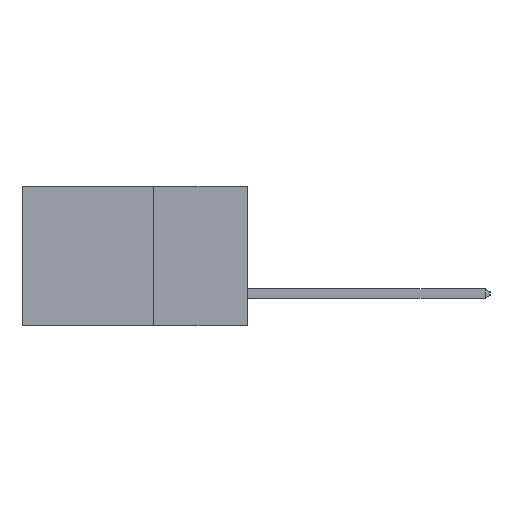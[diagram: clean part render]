
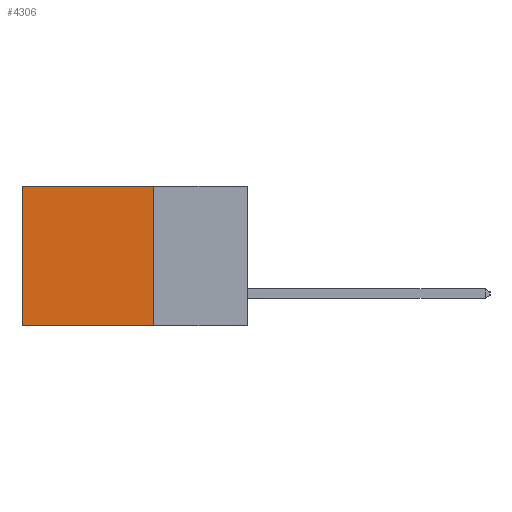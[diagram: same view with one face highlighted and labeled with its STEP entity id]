
A CAD part, left-side view. The second image highlights one B-rep face of the part: STEP entity #4306.
In plain terms, the highlighted planar face has unit normal (-1, 0, 0).
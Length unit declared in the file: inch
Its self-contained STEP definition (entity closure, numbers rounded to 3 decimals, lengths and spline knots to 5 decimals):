
#258 = FACE_OUTER_BOUND ( 'NONE', #11294, .T. ) ;
#432 = ORIENTED_EDGE ( 'NONE', *, *, #4121, .T. ) ;
#557 = VECTOR ( 'NONE', #14478, 39.37008 ) ;
#993 = LINE ( 'NONE', #14467, #557 ) ;
#1541 = VERTEX_POINT ( 'NONE', #5240 ) ;
#1829 = VECTOR ( 'NONE', #15657, 39.37008 ) ;
#1896 = CARTESIAN_POINT ( 'NONE',  ( 0.298, 0.25, 0. ) ) ;
#2650 = CARTESIAN_POINT ( 'NONE',  ( 0.298, 0.6, -0.37 ) ) ;
#3651 = VERTEX_POINT ( 'NONE', #2650 ) ;
#3961 = EDGE_CURVE ( 'NONE', #1541, #5538, #9149, .T. ) ;
#4121 = EDGE_CURVE ( 'NONE', #1541, #4907, #9777, .T. ) ;
#4306 = ADVANCED_FACE ( 'NONE', ( #258 ), #14654, .F. ) ;
#4907 = VERTEX_POINT ( 'NONE', #16112 ) ;
#4939 = VECTOR ( 'NONE', #8704, 39.37008 ) ;
#5240 = CARTESIAN_POINT ( 'NONE',  ( 0.298, 0.25, 0. ) ) ;
#5258 = EDGE_CURVE ( 'NONE', #5538, #3651, #12749, .T. ) ;
#5538 = VERTEX_POINT ( 'NONE', #16472 ) ;
#5621 = ORIENTED_EDGE ( 'NONE', *, *, #5258, .F. ) ;
#6092 = VECTOR ( 'NONE', #14406, 39.37008 ) ;
#6339 = EDGE_CURVE ( 'NONE', #4907, #3651, #993, .T. ) ;
#7039 = AXIS2_PLACEMENT_3D ( 'NONE', #8449, #14758, #12980 ) ;
#7514 = ORIENTED_EDGE ( 'NONE', *, *, #6339, .T. ) ;
#8449 = CARTESIAN_POINT ( 'NONE',  ( 0.298, 0.25, 0. ) ) ;
#8704 = DIRECTION ( 'NONE',  ( 0., 1., 0. ) ) ;
#9149 = LINE ( 'NONE', #16327, #1829 ) ;
#9777 = LINE ( 'NONE', #1896, #6092 ) ;
#11294 = EDGE_LOOP ( 'NONE', ( #7514, #5621, #14216, #432 ) ) ;
#12749 = LINE ( 'NONE', #13396, #4939 ) ;
#12980 = DIRECTION ( 'NONE',  ( 0., 0., -1. ) ) ;
#13396 = CARTESIAN_POINT ( 'NONE',  ( 0.298, 0.25, -0.37 ) ) ;
#14216 = ORIENTED_EDGE ( 'NONE', *, *, #3961, .F. ) ;
#14406 = DIRECTION ( 'NONE',  ( 0., 1., 0. ) ) ;
#14467 = CARTESIAN_POINT ( 'NONE',  ( 0.298, 0.6, 0. ) ) ;
#14478 = DIRECTION ( 'NONE',  ( 0., 0., -1. ) ) ;
#14654 = PLANE ( 'NONE',  #7039 ) ;
#14758 = DIRECTION ( 'NONE',  ( 1., 0., 0. ) ) ;
#15657 = DIRECTION ( 'NONE',  ( 0., 0., -1. ) ) ;
#16112 = CARTESIAN_POINT ( 'NONE',  ( 0.298, 0.6, 0. ) ) ;
#16327 = CARTESIAN_POINT ( 'NONE',  ( 0.298, 0.25, 0. ) ) ;
#16472 = CARTESIAN_POINT ( 'NONE',  ( 0.298, 0.25, -0.37 ) ) ;
